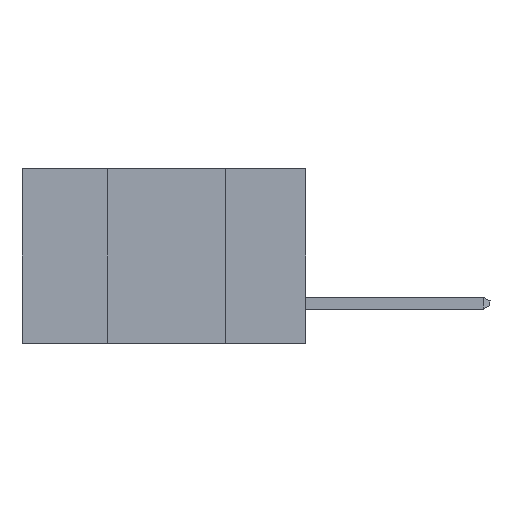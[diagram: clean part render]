
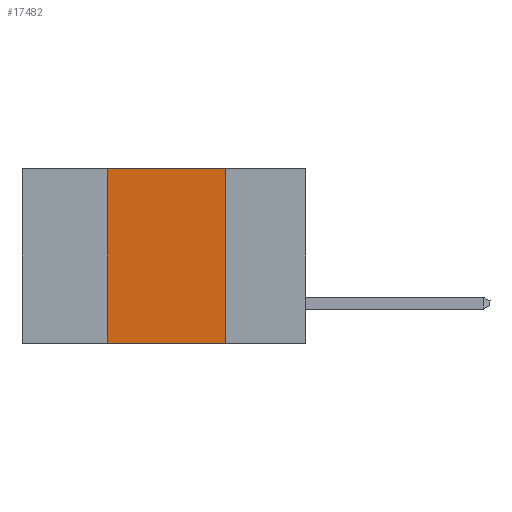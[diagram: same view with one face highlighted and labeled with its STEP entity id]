
A CAD part, left-side view. The second image highlights one B-rep face of the part: STEP entity #17482.
In plain terms, the highlighted planar face has unit normal (-1, 0, 0).
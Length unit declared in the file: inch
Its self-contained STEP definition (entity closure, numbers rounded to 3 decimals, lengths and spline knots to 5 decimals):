
#1238 = EDGE_CURVE ( 'NONE', #18516, #8496, #2051, .T. ) ;
#1313 = VECTOR ( 'NONE', #4606, 39.37008 ) ;
#2051 = LINE ( 'NONE', #10503, #1313 ) ;
#2670 = ORIENTED_EDGE ( 'NONE', *, *, #1238, .F. ) ;
#3137 = ORIENTED_EDGE ( 'NONE', *, *, #21918, .F. ) ;
#3351 = VECTOR ( 'NONE', #18307, 39.37008 ) ;
#3565 = EDGE_LOOP ( 'NONE', ( #3137, #2670, #22022, #16370 ) ) ;
#3992 = EDGE_CURVE ( 'NONE', #5218, #18516, #18853, .T. ) ;
#4606 = DIRECTION ( 'NONE',  ( 0., -1., 0. ) ) ;
#4905 = AXIS2_PLACEMENT_3D ( 'NONE', #7415, #5215, #20883 ) ;
#5215 = DIRECTION ( 'NONE',  ( 1., 0., 0. ) ) ;
#5218 = VERTEX_POINT ( 'NONE', #16669 ) ;
#5487 = FACE_OUTER_BOUND ( 'NONE', #3565, .T. ) ;
#5870 = VECTOR ( 'NONE', #23100, 39.37008 ) ;
#7415 = CARTESIAN_POINT ( 'NONE',  ( 0., 0.6, 0. ) ) ;
#8496 = VERTEX_POINT ( 'NONE', #16792 ) ;
#9881 = EDGE_CURVE ( 'NONE', #5218, #19931, #23821, .T. ) ;
#10503 = CARTESIAN_POINT ( 'NONE',  ( 0., 0.6, 0. ) ) ;
#10994 = CARTESIAN_POINT ( 'NONE',  ( 0., 0.42, -0.37 ) ) ;
#12723 = LINE ( 'NONE', #19394, #5870 ) ;
#13306 = DIRECTION ( 'NONE',  ( 0., 0., 1. ) ) ;
#15984 = CARTESIAN_POINT ( 'NONE',  ( 0., 0.6, -0.37 ) ) ;
#16370 = ORIENTED_EDGE ( 'NONE', *, *, #9881, .T. ) ;
#16669 = CARTESIAN_POINT ( 'NONE',  ( 0., 0.42, -0.37 ) ) ;
#16777 = PLANE ( 'NONE',  #4905 ) ;
#16792 = CARTESIAN_POINT ( 'NONE',  ( 0., 0.17, 0. ) ) ;
#17007 = CARTESIAN_POINT ( 'NONE',  ( 0., 0.42, 0. ) ) ;
#17169 = VECTOR ( 'NONE', #13306, 39.37008 ) ;
#17482 = ADVANCED_FACE ( 'NONE', ( #5487 ), #16777, .F. ) ;
#18029 = CARTESIAN_POINT ( 'NONE',  ( 0., 0.17, -0.37 ) ) ;
#18307 = DIRECTION ( 'NONE',  ( 0., -1., 0. ) ) ;
#18516 = VERTEX_POINT ( 'NONE', #17007 ) ;
#18853 = LINE ( 'NONE', #10994, #17169 ) ;
#19394 = CARTESIAN_POINT ( 'NONE',  ( 0., 0.17, -0.37 ) ) ;
#19931 = VERTEX_POINT ( 'NONE', #18029 ) ;
#20883 = DIRECTION ( 'NONE',  ( 0., 0., -1. ) ) ;
#21918 = EDGE_CURVE ( 'NONE', #8496, #19931, #12723, .T. ) ;
#22022 = ORIENTED_EDGE ( 'NONE', *, *, #3992, .F. ) ;
#23100 = DIRECTION ( 'NONE',  ( 0., 0., -1. ) ) ;
#23821 = LINE ( 'NONE', #15984, #3351 ) ;
